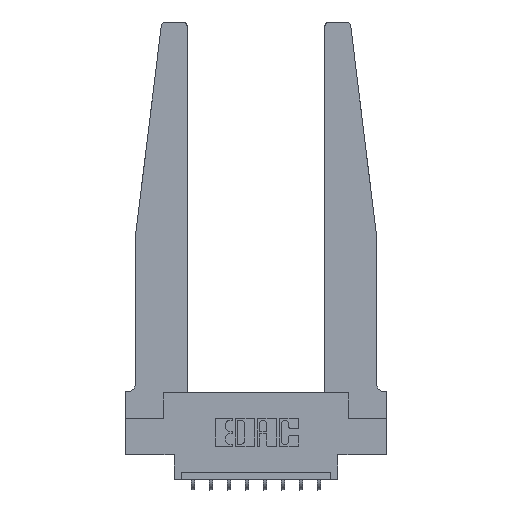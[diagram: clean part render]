
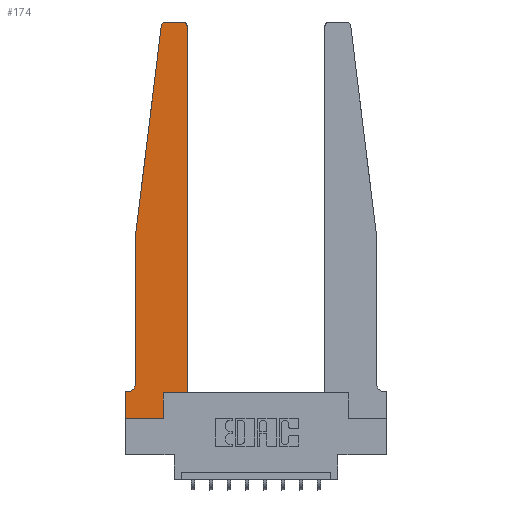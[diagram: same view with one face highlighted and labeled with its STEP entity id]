
A CAD part, top view. The second image highlights one B-rep face of the part: STEP entity #174.
In plain terms, the highlighted planar face has unit normal (0, 0, 1).
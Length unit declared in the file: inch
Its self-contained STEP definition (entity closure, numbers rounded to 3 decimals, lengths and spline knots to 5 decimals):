
#172 = DIRECTION ( 'NONE',  ( 1., 0., 0. ) ) ;
#174 = ADVANCED_FACE ( 'NONE', ( #11993 ), #4673, .T. ) ;
#267 = AXIS2_PLACEMENT_3D ( 'NONE', #11363, #6919, #172 ) ;
#287 = ORIENTED_EDGE ( 'NONE', *, *, #7390, .T. ) ;
#373 = CARTESIAN_POINT ( 'NONE',  ( 0.065, 1.25, 0.37 ) ) ;
#646 = VERTEX_POINT ( 'NONE', #14393 ) ;
#749 = EDGE_CURVE ( 'NONE', #8710, #3683, #9886, .T. ) ;
#841 = CARTESIAN_POINT ( 'NONE',  ( 0., 0.1875, 0.37 ) ) ;
#1051 = VECTOR ( 'NONE', #10902, 39.37008 ) ;
#2124 = VECTOR ( 'NONE', #5027, 39.37008 ) ;
#2320 = DIRECTION ( 'NONE',  ( 0., 0., 1. ) ) ;
#2619 = CARTESIAN_POINT ( 'NONE',  ( 0.425, 2.72, 0.37 ) ) ;
#3054 = VERTEX_POINT ( 'NONE', #2619 ) ;
#3215 = DIRECTION ( 'NONE',  ( -0.122, -0.992, 0. ) ) ;
#3509 = VERTEX_POINT ( 'NONE', #4609 ) ;
#3661 = ORIENTED_EDGE ( 'NONE', *, *, #5766, .T. ) ;
#3683 = VERTEX_POINT ( 'NONE', #9373 ) ;
#3760 = LINE ( 'NONE', #4831, #9720 ) ;
#3790 = VECTOR ( 'NONE', #6917, 39.37008 ) ;
#3800 = VECTOR ( 'NONE', #3215, 39.37008 ) ;
#3981 = VERTEX_POINT ( 'NONE', #841 ) ;
#4093 = LINE ( 'NONE', #8676, #1051 ) ;
#4377 = ORIENTED_EDGE ( 'NONE', *, *, #10304, .T. ) ;
#4459 = CIRCLE ( 'NONE', #9844, 0.03 ) ;
#4609 = CARTESIAN_POINT ( 'NONE',  ( 0.015, 0.1875, 0.37 ) ) ;
#4673 = PLANE ( 'NONE',  #267 ) ;
#4773 = EDGE_CURVE ( 'NONE', #3683, #5662, #6412, .T. ) ;
#4814 = CARTESIAN_POINT ( 'NONE',  ( 0.25, 2.75, 0.37 ) ) ;
#4825 = DIRECTION ( 'NONE',  ( 0., 0., -1. ) ) ;
#4831 = CARTESIAN_POINT ( 'NONE',  ( 0., 0., 0.37 ) ) ;
#4873 = EDGE_CURVE ( 'NONE', #9911, #13213, #13920, .T. ) ;
#4888 = CARTESIAN_POINT ( 'NONE',  ( 0.395, 2.72, 0.37 ) ) ;
#4913 = VERTEX_POINT ( 'NONE', #373 ) ;
#4974 = CARTESIAN_POINT ( 'NONE',  ( 0., 0., 0.37 ) ) ;
#5027 = DIRECTION ( 'NONE',  ( 1., 0., 0. ) ) ;
#5490 = VECTOR ( 'NONE', #13360, 39.37008 ) ;
#5662 = VERTEX_POINT ( 'NONE', #13382 ) ;
#5709 = EDGE_CURVE ( 'NONE', #13213, #646, #4459, .T. ) ;
#5766 = EDGE_CURVE ( 'NONE', #3981, #7831, #3760, .T. ) ;
#5835 = LINE ( 'NONE', #6664, #5490 ) ;
#6018 = DIRECTION ( 'NONE',  ( 1., 0., 0. ) ) ;
#6397 = CARTESIAN_POINT ( 'NONE',  ( 0.065, 0.2375, 0.37 ) ) ;
#6412 = LINE ( 'NONE', #13608, #3790 ) ;
#6441 = ORIENTED_EDGE ( 'NONE', *, *, #749, .T. ) ;
#6576 = CARTESIAN_POINT ( 'NONE',  ( 0.065, 1.25, 0.37 ) ) ;
#6594 = EDGE_LOOP ( 'NONE', ( #8797, #7940, #14343, #10787, #6914, #12171, #3661, #9760, #6441, #14025, #287, #4377 ) ) ;
#6664 = CARTESIAN_POINT ( 'NONE',  ( 0.065, 0.1875, 0.37 ) ) ;
#6755 = DIRECTION ( 'NONE',  ( 0., 1., 0. ) ) ;
#6841 = EDGE_CURVE ( 'NONE', #3509, #3981, #5835, .T. ) ;
#6914 = ORIENTED_EDGE ( 'NONE', *, *, #7732, .T. ) ;
#6917 = DIRECTION ( 'NONE',  ( 1., 0., 0. ) ) ;
#6919 = DIRECTION ( 'NONE',  ( 0., 0., 1. ) ) ;
#7390 = EDGE_CURVE ( 'NONE', #5662, #3054, #4093, .T. ) ;
#7431 = AXIS2_PLACEMENT_3D ( 'NONE', #4888, #12719, #6018 ) ;
#7621 = CARTESIAN_POINT ( 'NONE',  ( 0.065, 1.25, 0.37 ) ) ;
#7732 = EDGE_CURVE ( 'NONE', #7984, #3509, #14046, .T. ) ;
#7796 = EDGE_CURVE ( 'NONE', #7831, #8710, #10723, .T. ) ;
#7831 = VERTEX_POINT ( 'NONE', #10592 ) ;
#7940 = ORIENTED_EDGE ( 'NONE', *, *, #5709, .T. ) ;
#7975 = DIRECTION ( 'NONE',  ( 0., -1., 0. ) ) ;
#7984 = VERTEX_POINT ( 'NONE', #6397 ) ;
#8132 = CARTESIAN_POINT ( 'NONE',  ( 0.27653, 2.75, 0.37 ) ) ;
#8676 = CARTESIAN_POINT ( 'NONE',  ( 0.425, 0.18, 0.37 ) ) ;
#8710 = VERTEX_POINT ( 'NONE', #10371 ) ;
#8797 = ORIENTED_EDGE ( 'NONE', *, *, #4873, .T. ) ;
#9059 = CARTESIAN_POINT ( 'NONE',  ( 0.27653, 2.72, 0.37 ) ) ;
#9373 = CARTESIAN_POINT ( 'NONE',  ( 0.2605, 0.18, 0.37 ) ) ;
#9720 = VECTOR ( 'NONE', #7975, 39.37008 ) ;
#9760 = ORIENTED_EDGE ( 'NONE', *, *, #7796, .T. ) ;
#9844 = AXIS2_PLACEMENT_3D ( 'NONE', #9059, #2320, #10165 ) ;
#9886 = LINE ( 'NONE', #11298, #12849 ) ;
#9911 = VERTEX_POINT ( 'NONE', #12781 ) ;
#10165 = DIRECTION ( 'NONE',  ( 1., 0., 0. ) ) ;
#10304 = EDGE_CURVE ( 'NONE', #3054, #9911, #11898, .T. ) ;
#10371 = CARTESIAN_POINT ( 'NONE',  ( 0.2605, 0., 0.37 ) ) ;
#10592 = CARTESIAN_POINT ( 'NONE',  ( 0., 0., 0.37 ) ) ;
#10723 = LINE ( 'NONE', #4974, #2124 ) ;
#10787 = ORIENTED_EDGE ( 'NONE', *, *, #12460, .T. ) ;
#10902 = DIRECTION ( 'NONE',  ( 0., 1., 0. ) ) ;
#10950 = VECTOR ( 'NONE', #12641, 39.37008 ) ;
#11298 = CARTESIAN_POINT ( 'NONE',  ( 0.2605, 0.18, 0.37 ) ) ;
#11363 = CARTESIAN_POINT ( 'NONE',  ( 0., 0.1875, 0.37 ) ) ;
#11519 = CARTESIAN_POINT ( 'NONE',  ( 0.015, 0.2375, 0.37 ) ) ;
#11898 = CIRCLE ( 'NONE', #7431, 0.03 ) ;
#11993 = FACE_OUTER_BOUND ( 'NONE', #6594, .T. ) ;
#12171 = ORIENTED_EDGE ( 'NONE', *, *, #6841, .T. ) ;
#12210 = VECTOR ( 'NONE', #13186, 39.37008 ) ;
#12460 = EDGE_CURVE ( 'NONE', #4913, #7984, #12567, .T. ) ;
#12567 = LINE ( 'NONE', #7621, #12210 ) ;
#12641 = DIRECTION ( 'NONE',  ( -1., 0., 0. ) ) ;
#12653 = AXIS2_PLACEMENT_3D ( 'NONE', #11519, #4825, #12657 ) ;
#12657 = DIRECTION ( 'NONE',  ( -1., 0., 0. ) ) ;
#12715 = LINE ( 'NONE', #6576, #3800 ) ;
#12719 = DIRECTION ( 'NONE',  ( 0., 0., 1. ) ) ;
#12781 = CARTESIAN_POINT ( 'NONE',  ( 0.395, 2.75, 0.37 ) ) ;
#12849 = VECTOR ( 'NONE', #6755, 39.37008 ) ;
#13179 = EDGE_CURVE ( 'NONE', #646, #4913, #12715, .T. ) ;
#13186 = DIRECTION ( 'NONE',  ( 0., -1., 0. ) ) ;
#13213 = VERTEX_POINT ( 'NONE', #8132 ) ;
#13360 = DIRECTION ( 'NONE',  ( -1., 0., 0. ) ) ;
#13382 = CARTESIAN_POINT ( 'NONE',  ( 0.425, 0.18, 0.37 ) ) ;
#13608 = CARTESIAN_POINT ( 'NONE',  ( 0.425, 0.18, 0.37 ) ) ;
#13920 = LINE ( 'NONE', #4814, #10950 ) ;
#14025 = ORIENTED_EDGE ( 'NONE', *, *, #4773, .T. ) ;
#14046 = CIRCLE ( 'NONE', #12653, 0.05 ) ;
#14343 = ORIENTED_EDGE ( 'NONE', *, *, #13179, .T. ) ;
#14393 = CARTESIAN_POINT ( 'NONE',  ( 0.24675, 2.72367, 0.37 ) ) ;
